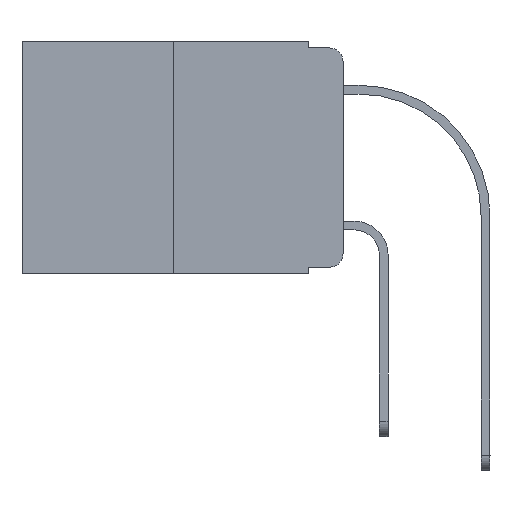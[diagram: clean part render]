
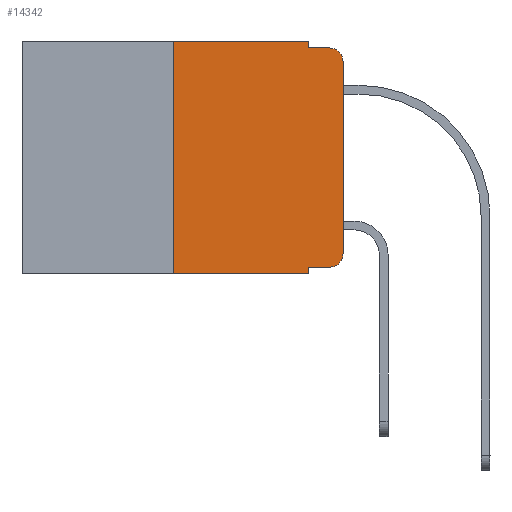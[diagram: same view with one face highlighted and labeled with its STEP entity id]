
A CAD part, left-side view. The second image highlights one B-rep face of the part: STEP entity #14342.
In plain terms, the highlighted planar face has unit normal (-1, 0, 0).
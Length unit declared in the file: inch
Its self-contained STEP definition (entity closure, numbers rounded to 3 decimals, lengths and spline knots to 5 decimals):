
#349 = VERTEX_POINT ( 'NONE', #9884 ) ;
#358 = DIRECTION ( 'NONE',  ( 0., -1., 0. ) ) ;
#1485 = EDGE_CURVE ( 'NONE', #10445, #7012, #15625, .T. ) ;
#1545 = VERTEX_POINT ( 'NONE', #14673 ) ;
#1909 = VERTEX_POINT ( 'NONE', #15380 ) ;
#1942 = ORIENTED_EDGE ( 'NONE', *, *, #16876, .F. ) ;
#1992 = LINE ( 'NONE', #12704, #3276 ) ;
#2817 = ORIENTED_EDGE ( 'NONE', *, *, #17032, .F. ) ;
#3033 = LINE ( 'NONE', #15511, #4831 ) ;
#3080 = CIRCLE ( 'NONE', #10831, 0.02 ) ;
#3276 = VECTOR ( 'NONE', #358, 39.37008 ) ;
#3479 = VECTOR ( 'NONE', #11573, 39.37008 ) ;
#3492 = ORIENTED_EDGE ( 'NONE', *, *, #12143, .T. ) ;
#3640 = CARTESIAN_POINT ( 'NONE',  ( 0., 0., -0.03 ) ) ;
#3724 = VERTEX_POINT ( 'NONE', #6562 ) ;
#3763 = CARTESIAN_POINT ( 'NONE',  ( 0., 0.051, 0. ) ) ;
#4705 = EDGE_CURVE ( 'NONE', #12906, #7012, #10109, .T. ) ;
#4831 = VECTOR ( 'NONE', #8689, 39.37008 ) ;
#5093 = EDGE_CURVE ( 'NONE', #11316, #13248, #3080, .T. ) ;
#5100 = ORIENTED_EDGE ( 'NONE', *, *, #14275, .F. ) ;
#6108 = EDGE_CURVE ( 'NONE', #1909, #3724, #14962, .T. ) ;
#6322 = DIRECTION ( 'NONE',  ( 0., 0., -1. ) ) ;
#6382 = EDGE_CURVE ( 'NONE', #1545, #11316, #10262, .T. ) ;
#6529 = ORIENTED_EDGE ( 'NONE', *, *, #4705, .F. ) ;
#6562 = CARTESIAN_POINT ( 'NONE',  ( 0., 0.25, 0. ) ) ;
#7012 = VERTEX_POINT ( 'NONE', #13460 ) ;
#7224 = EDGE_CURVE ( 'NONE', #13248, #10445, #3033, .T. ) ;
#7272 = CARTESIAN_POINT ( 'NONE',  ( 0., 0.051, 0. ) ) ;
#7425 = VECTOR ( 'NONE', #7659, 39.37008 ) ;
#7628 = DIRECTION ( 'NONE',  ( -1., 0., 0. ) ) ;
#7659 = DIRECTION ( 'NONE',  ( 0., -1., 0. ) ) ;
#7667 = DIRECTION ( 'NONE',  ( 0., -1., 0. ) ) ;
#8047 = CARTESIAN_POINT ( 'NONE',  ( 0., 0.25, 0. ) ) ;
#8223 = ORIENTED_EDGE ( 'NONE', *, *, #6382, .T. ) ;
#8281 = AXIS2_PLACEMENT_3D ( 'NONE', #10185, #15667, #6322 ) ;
#8689 = DIRECTION ( 'NONE',  ( 0., 0., 1. ) ) ;
#8767 = CARTESIAN_POINT ( 'NONE',  ( 0., 0.051, 0. ) ) ;
#8789 = LINE ( 'NONE', #7272, #3479 ) ;
#8906 = CARTESIAN_POINT ( 'NONE',  ( 0., 0.02, -0.333 ) ) ;
#8918 = VECTOR ( 'NONE', #10546, 39.37008 ) ;
#9281 = CARTESIAN_POINT ( 'NONE',  ( 0., 0., -0.313 ) ) ;
#9884 = CARTESIAN_POINT ( 'NONE',  ( 0., 0.051, -0.343 ) ) ;
#10109 = LINE ( 'NONE', #17019, #11783 ) ;
#10185 = CARTESIAN_POINT ( 'NONE',  ( 0., 0.473, 0. ) ) ;
#10219 = LINE ( 'NONE', #3763, #16916 ) ;
#10239 = VERTEX_POINT ( 'NONE', #8767 ) ;
#10262 = LINE ( 'NONE', #14302, #11754 ) ;
#10445 = VERTEX_POINT ( 'NONE', #3640 ) ;
#10546 = DIRECTION ( 'NONE',  ( 0., 0., 1. ) ) ;
#10831 = AXIS2_PLACEMENT_3D ( 'NONE', #11854, #7628, #14458 ) ;
#11316 = VERTEX_POINT ( 'NONE', #8906 ) ;
#11535 = CARTESIAN_POINT ( 'NONE',  ( 0., 0.473, 0. ) ) ;
#11573 = DIRECTION ( 'NONE',  ( 0., 0., -1. ) ) ;
#11705 = LINE ( 'NONE', #11535, #7425 ) ;
#11754 = VECTOR ( 'NONE', #14127, 39.37008 ) ;
#11783 = VECTOR ( 'NONE', #7667, 39.37008 ) ;
#11805 = DIRECTION ( 'NONE',  ( 0., 0., -1. ) ) ;
#11854 = CARTESIAN_POINT ( 'NONE',  ( 0., 0.02, -0.313 ) ) ;
#12143 = EDGE_CURVE ( 'NONE', #1909, #349, #1992, .T. ) ;
#12704 = CARTESIAN_POINT ( 'NONE',  ( 0., 0.473, -0.343 ) ) ;
#12707 = ORIENTED_EDGE ( 'NONE', *, *, #7224, .T. ) ;
#12906 = VERTEX_POINT ( 'NONE', #16485 ) ;
#13143 = PLANE ( 'NONE',  #8281 ) ;
#13239 = ORIENTED_EDGE ( 'NONE', *, *, #5093, .T. ) ;
#13248 = VERTEX_POINT ( 'NONE', #9281 ) ;
#13460 = CARTESIAN_POINT ( 'NONE',  ( 0., 0.02, -0.01 ) ) ;
#13727 = EDGE_LOOP ( 'NONE', ( #12707, #15038, #6529, #2817, #5100, #14503, #3492, #1942, #8223, #13239 ) ) ;
#14127 = DIRECTION ( 'NONE',  ( 0., -1., 0. ) ) ;
#14275 = EDGE_CURVE ( 'NONE', #3724, #10239, #11705, .T. ) ;
#14302 = CARTESIAN_POINT ( 'NONE',  ( 0., 0.051, -0.333 ) ) ;
#14310 = FACE_OUTER_BOUND ( 'NONE', #13727, .T. ) ;
#14342 = ADVANCED_FACE ( 'NONE', ( #14310 ), #13143, .F. ) ;
#14458 = DIRECTION ( 'NONE',  ( 0., 0., -1. ) ) ;
#14495 = CARTESIAN_POINT ( 'NONE',  ( 0., 0.02, -0.03 ) ) ;
#14503 = ORIENTED_EDGE ( 'NONE', *, *, #6108, .F. ) ;
#14673 = CARTESIAN_POINT ( 'NONE',  ( 0., 0.051, -0.333 ) ) ;
#14962 = LINE ( 'NONE', #8047, #8918 ) ;
#15038 = ORIENTED_EDGE ( 'NONE', *, *, #1485, .T. ) ;
#15380 = CARTESIAN_POINT ( 'NONE',  ( 0., 0.25, -0.343 ) ) ;
#15511 = CARTESIAN_POINT ( 'NONE',  ( 0., 0., 0. ) ) ;
#15625 = CIRCLE ( 'NONE', #15893, 0.02 ) ;
#15667 = DIRECTION ( 'NONE',  ( 1., 0., 0. ) ) ;
#15893 = AXIS2_PLACEMENT_3D ( 'NONE', #14495, #17553, #11805 ) ;
#16048 = DIRECTION ( 'NONE',  ( 0., 0., -1. ) ) ;
#16485 = CARTESIAN_POINT ( 'NONE',  ( 0., 0.051, -0.01 ) ) ;
#16876 = EDGE_CURVE ( 'NONE', #1545, #349, #8789, .T. ) ;
#16916 = VECTOR ( 'NONE', #16048, 39.37008 ) ;
#17019 = CARTESIAN_POINT ( 'NONE',  ( 0., 0.051, -0.01 ) ) ;
#17032 = EDGE_CURVE ( 'NONE', #10239, #12906, #10219, .T. ) ;
#17553 = DIRECTION ( 'NONE',  ( -1., 0., 0. ) ) ;
